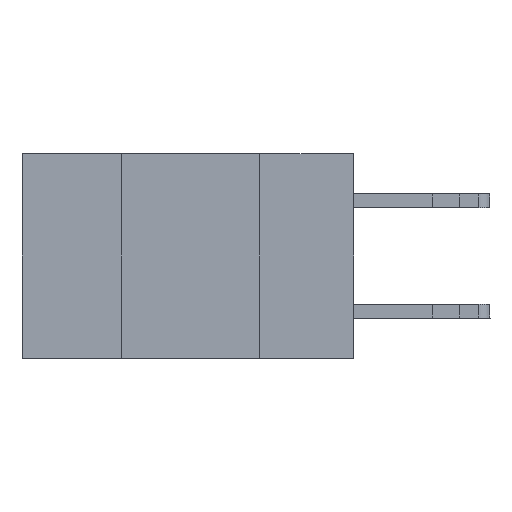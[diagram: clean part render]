
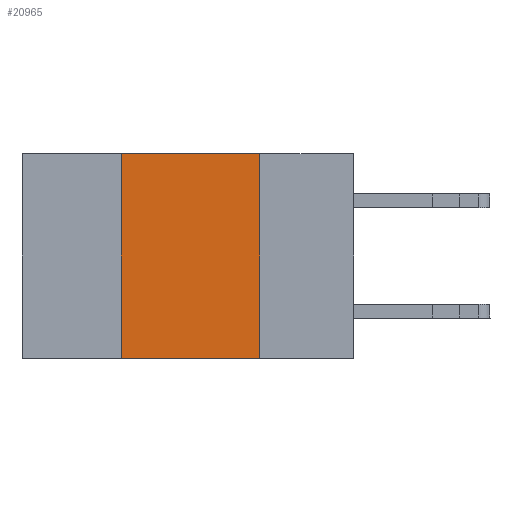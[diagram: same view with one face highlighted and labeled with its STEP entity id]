
A CAD part, left-side view. The second image highlights one B-rep face of the part: STEP entity #20965.
In plain terms, the highlighted planar face has unit normal (-1, 0, 0).
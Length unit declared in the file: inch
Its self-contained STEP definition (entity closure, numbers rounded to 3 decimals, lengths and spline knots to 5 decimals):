
#10 = VERTEX_POINT ( 'NONE', #14747 ) ;
#145 = CARTESIAN_POINT ( 'NONE',  ( 0., 0.6, 0. ) ) ;
#794 = CARTESIAN_POINT ( 'NONE',  ( 0., 0.6, -0.37 ) ) ;
#1069 = EDGE_CURVE ( 'NONE', #20406, #10, #18236, .T. ) ;
#2345 = CARTESIAN_POINT ( 'NONE',  ( 0., 0.6, 0. ) ) ;
#2809 = VECTOR ( 'NONE', #16805, 39.37008 ) ;
#4189 = VERTEX_POINT ( 'NONE', #5581 ) ;
#4569 = FACE_OUTER_BOUND ( 'NONE', #21543, .T. ) ;
#4615 = CARTESIAN_POINT ( 'NONE',  ( 0., 0.42, 0. ) ) ;
#5581 = CARTESIAN_POINT ( 'NONE',  ( 0., 0.42, 0. ) ) ;
#6471 = DIRECTION ( 'NONE',  ( 0., 0., 1. ) ) ;
#6508 = CARTESIAN_POINT ( 'NONE',  ( 0., 0.17, 0. ) ) ;
#6574 = VERTEX_POINT ( 'NONE', #21900 ) ;
#7692 = DIRECTION ( 'NONE',  ( 1., 0., 0. ) ) ;
#9760 = VECTOR ( 'NONE', #6471, 39.37008 ) ;
#9919 = ORIENTED_EDGE ( 'NONE', *, *, #1069, .F. ) ;
#10052 = ORIENTED_EDGE ( 'NONE', *, *, #21032, .F. ) ;
#10094 = ORIENTED_EDGE ( 'NONE', *, *, #10272, .F. ) ;
#10141 = ORIENTED_EDGE ( 'NONE', *, *, #17467, .T. ) ;
#10272 = EDGE_CURVE ( 'NONE', #6574, #4189, #19324, .T. ) ;
#13166 = LINE ( 'NONE', #794, #22876 ) ;
#13452 = DIRECTION ( 'NONE',  ( 0., 0., -1. ) ) ;
#13528 = DIRECTION ( 'NONE',  ( 0., -1., 0. ) ) ;
#14692 = CARTESIAN_POINT ( 'NONE',  ( 0., 0.17, 0. ) ) ;
#14747 = CARTESIAN_POINT ( 'NONE',  ( 0., 0.17, -0.37 ) ) ;
#16570 = PLANE ( 'NONE',  #20936 ) ;
#16805 = DIRECTION ( 'NONE',  ( 0., -1., 0. ) ) ;
#17467 = EDGE_CURVE ( 'NONE', #6574, #10, #13166, .T. ) ;
#18236 = LINE ( 'NONE', #6508, #22580 ) ;
#19324 = LINE ( 'NONE', #4615, #9760 ) ;
#20257 = DIRECTION ( 'NONE',  ( 0., 0., -1. ) ) ;
#20406 = VERTEX_POINT ( 'NONE', #14692 ) ;
#20936 = AXIS2_PLACEMENT_3D ( 'NONE', #145, #7692, #20257 ) ;
#20965 = ADVANCED_FACE ( 'NONE', ( #4569 ), #16570, .F. ) ;
#21032 = EDGE_CURVE ( 'NONE', #4189, #20406, #22153, .T. ) ;
#21543 = EDGE_LOOP ( 'NONE', ( #9919, #10052, #10094, #10141 ) ) ;
#21900 = CARTESIAN_POINT ( 'NONE',  ( 0., 0.42, -0.37 ) ) ;
#22153 = LINE ( 'NONE', #2345, #2809 ) ;
#22580 = VECTOR ( 'NONE', #13452, 39.37008 ) ;
#22876 = VECTOR ( 'NONE', #13528, 39.37008 ) ;
